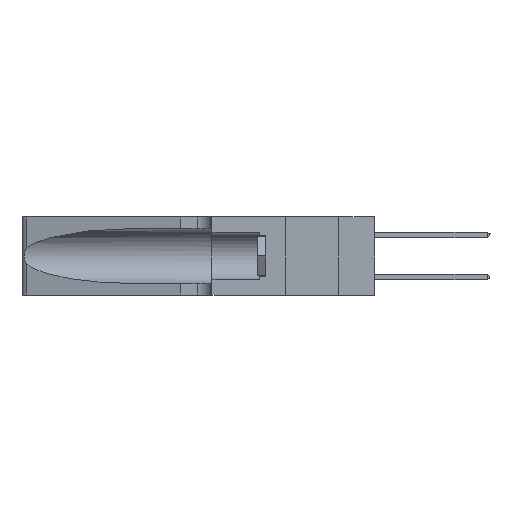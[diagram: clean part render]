
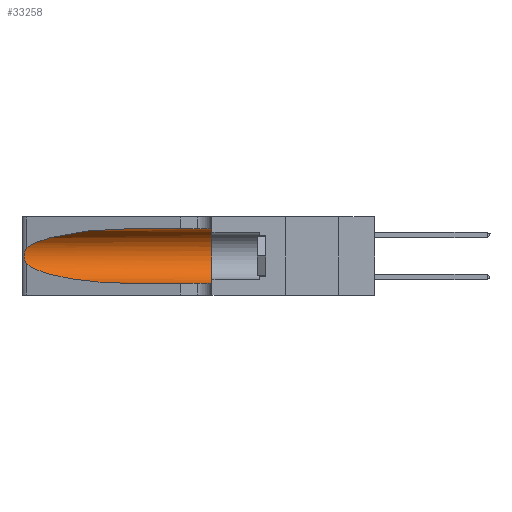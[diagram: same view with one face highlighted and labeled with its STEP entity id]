
A CAD part, left-side view. The second image highlights one B-rep face of the part: STEP entity #33258.
In plain terms, the highlighted cylindrical face has radius 3.308 mm (diameter 6.617 mm), a partial arc.
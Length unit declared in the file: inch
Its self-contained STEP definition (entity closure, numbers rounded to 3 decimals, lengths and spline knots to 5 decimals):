
#714 = ORIENTED_EDGE ( 'NONE', *, *, #36783, .T. ) ;
#879 = DIRECTION ( 'NONE',  ( 0., 0., -1. ) ) ;
#1355 = CARTESIAN_POINT ( 'NONE',  ( 0.1305, 1.61858, 0.31525 ) ) ;
#1899 = CARTESIAN_POINT ( 'NONE',  ( 0.25639, 1.23184, 0.21858 ) ) ;
#2495 = CARTESIAN_POINT ( 'NONE',  ( 0.18966, 0.96281, 0.05475 ) ) ;
#3555 = DIRECTION ( 'NONE',  ( 0., 1., 0. ) ) ;
#4242 = CARTESIAN_POINT ( 'NONE',  ( 0.1305, 1.61858, 0.185 ) ) ;
#5058 = CARTESIAN_POINT ( 'NONE',  ( 0.1305, 1.61858, 0.05475 ) ) ;
#5418 = CARTESIAN_POINT ( 'NONE',  ( 0.25854, 1.2359, 0.20912 ) ) ;
#5820 = VERTEX_POINT ( 'NONE', #23026 ) ;
#6098 = ORIENTED_EDGE ( 'NONE', *, *, #6231, .F. ) ;
#6193 =( BOUNDED_CURVE ( )  B_SPLINE_CURVE ( 3, ( #40710, #23529, #2495, #26990 ),
 .UNSPECIFIED., .F., .T. ) 
 B_SPLINE_CURVE_WITH_KNOTS ( ( 4, 4 ),
 ( 3.44316, 4.71239 ),
 .UNSPECIFIED. ) 
 CURVE ( )  GEOMETRIC_REPRESENTATION_ITEM ( )  RATIONAL_B_SPLINE_CURVE ( ( 1., 0.87, 0.87, 1. ) ) 
 REPRESENTATION_ITEM ( '' )  );
#6231 = EDGE_CURVE ( 'NONE', #29597, #31536, #36466, .T. ) ;
#7061 = CARTESIAN_POINT ( 'NONE',  ( 0.1305, 0.72297, 0.31525 ) ) ;
#8098 = VECTOR ( 'NONE', #43344, 39.37008 ) ;
#8407 = DIRECTION ( 'NONE',  ( 0., -1., 0. ) ) ;
#8971 = CARTESIAN_POINT ( 'NONE',  ( 0.26075, 1.23896, 0.19203 ) ) ;
#10032 = AXIS2_PLACEMENT_3D ( 'NONE', #24572, #3555, #28025 ) ;
#10054 = CARTESIAN_POINT ( 'NONE',  ( 0.1305, 0.72297, 0.31525 ) ) ;
#10447 = EDGE_LOOP ( 'NONE', ( #32039, #28545, #38441, #714, #22375, #6098 ) ) ;
#12388 = CARTESIAN_POINT ( 'NONE',  ( 0.25487, 1.22718, 0.22369 ) ) ;
#12535 = CARTESIAN_POINT ( 'NONE',  ( 0.26017, 1.23833, 0.17102 ) ) ;
#13320 = EDGE_CURVE ( 'NONE', #31536, #15013, #16550, .T. ) ;
#13534 = FACE_OUTER_BOUND ( 'NONE', #10447, .T. ) ;
#13627 = CARTESIAN_POINT ( 'NONE',  ( 0.18966, 0.96281, 0.31525 ) ) ;
#14803 = VECTOR ( 'NONE', #8407, 39.37008 ) ;
#15013 = VERTEX_POINT ( 'NONE', #41940 ) ;
#15056 = CARTESIAN_POINT ( 'NONE',  ( 0.1305, 0.72297, 0.05475 ) ) ;
#16095 = CARTESIAN_POINT ( 'NONE',  ( 0.25487, 1.22718, 0.22369 ) ) ;
#16096 = CARTESIAN_POINT ( 'NONE',  ( 0.25789, 1.23486, 0.15765 ) ) ;
#16550 = CIRCLE ( 'NONE', #10032, 0.13025 ) ;
#18456 = DIRECTION ( 'NONE',  ( 0., -1., 0. ) ) ;
#19240 = VERTEX_POINT ( 'NONE', #15056 ) ;
#19618 = CARTESIAN_POINT ( 'NONE',  ( 0.25555, 1.22993, 0.14849 ) ) ;
#20688 = CARTESIAN_POINT ( 'NONE',  ( 0.25487, 1.22718, 0.22369 ) ) ;
#21752 = CYLINDRICAL_SURFACE ( 'NONE', #36995, 0.13025 ) ;
#21938 = EDGE_CURVE ( 'NONE', #5820, #19240, #6193, .T. ) ;
#22375 = ORIENTED_EDGE ( 'NONE', *, *, #13320, .F. ) ;
#23026 = CARTESIAN_POINT ( 'NONE',  ( 0.25487, 1.22718, 0.14631 ) ) ;
#23529 = CARTESIAN_POINT ( 'NONE',  ( 0.2373, 1.15595, 0.08982 ) ) ;
#24229 = CARTESIAN_POINT ( 'NONE',  ( 0.1305, 0.35, 0.31525 ) ) ;
#24572 = CARTESIAN_POINT ( 'NONE',  ( 0.1305, 0.35, 0.185 ) ) ;
#24581 = EDGE_CURVE ( 'NONE', #32127, #5820, #35237, .T. ) ;
#26399 = CARTESIAN_POINT ( 'NONE',  ( 0.25787, 1.23484, 0.2124 ) ) ;
#26717 = LINE ( 'NONE', #5058, #8098 ) ;
#26990 = CARTESIAN_POINT ( 'NONE',  ( 0.1305, 0.72297, 0.05475 ) ) ;
#27232 =( BOUNDED_CURVE ( )  B_SPLINE_CURVE ( 3, ( #10054, #13627, #41322, #20688 ),
 .UNSPECIFIED., .F., .F. ) 
 B_SPLINE_CURVE_WITH_KNOTS ( ( 4, 4 ),
 ( 1.5708, 2.84003 ),
 .UNSPECIFIED. ) 
 CURVE ( )  GEOMETRIC_REPRESENTATION_ITEM ( )  RATIONAL_B_SPLINE_CURVE ( ( 1., 0.87, 0.87, 1. ) ) 
 REPRESENTATION_ITEM ( '' )  );
#27558 = EDGE_CURVE ( 'NONE', #29597, #32127, #27232, .T. ) ;
#28025 = DIRECTION ( 'NONE',  ( 0., 0., 1. ) ) ;
#28545 = ORIENTED_EDGE ( 'NONE', *, *, #24581, .T. ) ;
#29597 = VERTEX_POINT ( 'NONE', #7061 ) ;
#29857 = CARTESIAN_POINT ( 'NONE',  ( 0.26018, 1.23835, 0.19895 ) ) ;
#31536 = VERTEX_POINT ( 'NONE', #24229 ) ;
#32039 = ORIENTED_EDGE ( 'NONE', *, *, #27558, .T. ) ;
#32127 = VERTEX_POINT ( 'NONE', #16095 ) ;
#33181 = CARTESIAN_POINT ( 'NONE',  ( 0.25555, 1.22994, 0.2215 ) ) ;
#33258 = ADVANCED_FACE ( 'NONE', ( #13534 ), #21752, .F. ) ;
#33330 = CARTESIAN_POINT ( 'NONE',  ( 0.26075, 1.23896, 0.178 ) ) ;
#35237 = B_SPLINE_CURVE_WITH_KNOTS ( 'NONE', 3,
 ( #12388, #33181, #1899, #26399, #5418, #29857, #8971, #33330, #12535, #36795, #16096, #40270, #19618, #43704 ),
 .UNSPECIFIED., .F., .F.,
 ( 4, 2, 2, 2, 2, 2, 4 ),
 ( 0., 0.00027, 0.00053, 0.00107, 0.0016, 0.00187, 0.00214 ),
 .UNSPECIFIED. ) ;
#36466 = LINE ( 'NONE', #1355, #14803 ) ;
#36783 = EDGE_CURVE ( 'NONE', #19240, #15013, #26717, .T. ) ;
#36795 = CARTESIAN_POINT ( 'NONE',  ( 0.25856, 1.23593, 0.16098 ) ) ;
#36995 = AXIS2_PLACEMENT_3D ( 'NONE', #4242, #18456, #879 ) ;
#38441 = ORIENTED_EDGE ( 'NONE', *, *, #21938, .T. ) ;
#40270 = CARTESIAN_POINT ( 'NONE',  ( 0.25639, 1.23186, 0.15144 ) ) ;
#40710 = CARTESIAN_POINT ( 'NONE',  ( 0.25487, 1.22718, 0.14631 ) ) ;
#41322 = CARTESIAN_POINT ( 'NONE',  ( 0.2373, 1.15595, 0.28018 ) ) ;
#41940 = CARTESIAN_POINT ( 'NONE',  ( 0.1305, 0.35, 0.05475 ) ) ;
#43344 = DIRECTION ( 'NONE',  ( 0., -1., 0. ) ) ;
#43704 = CARTESIAN_POINT ( 'NONE',  ( 0.25487, 1.22718, 0.14631 ) ) ;
